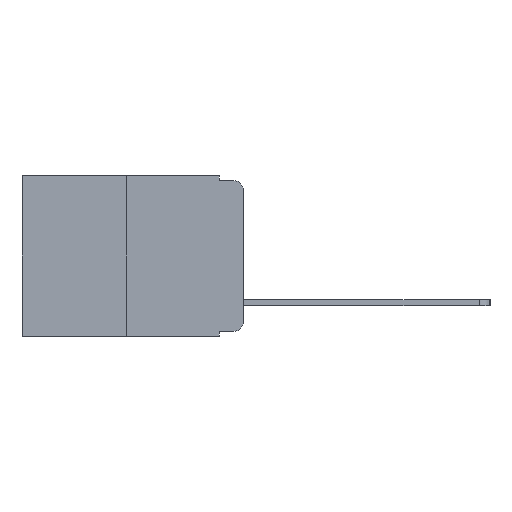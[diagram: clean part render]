
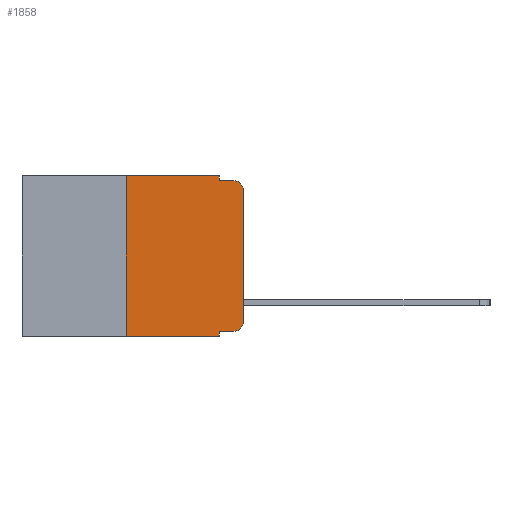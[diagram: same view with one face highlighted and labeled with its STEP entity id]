
A CAD part, left-side view. The second image highlights one B-rep face of the part: STEP entity #1858.
In plain terms, the highlighted planar face has unit normal (-1, 0, 0).
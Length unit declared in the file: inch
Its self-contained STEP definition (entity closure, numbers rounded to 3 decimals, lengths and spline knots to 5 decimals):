
#98 = DIRECTION ( 'NONE',  ( 0., 0., 1. ) ) ;
#257 = DIRECTION ( 'NONE',  ( 0., 0., -1. ) ) ;
#372 = CIRCLE ( 'NONE', #8661, 0.02 ) ;
#564 = DIRECTION ( 'NONE',  ( 0., 0., -1. ) ) ;
#1256 = EDGE_CURVE ( 'NONE', #14005, #2624, #5090, .T. ) ;
#1356 = DIRECTION ( 'NONE',  ( 0., 0., -1. ) ) ;
#1439 = CARTESIAN_POINT ( 'NONE',  ( 0., 0., -0.313 ) ) ;
#1517 = VERTEX_POINT ( 'NONE', #8939 ) ;
#1563 = AXIS2_PLACEMENT_3D ( 'NONE', #9882, #9736, #1356 ) ;
#1858 = ADVANCED_FACE ( 'NONE', ( #3646 ), #2925, .F. ) ;
#1863 = CIRCLE ( 'NONE', #1563, 0.02 ) ;
#1939 = AXIS2_PLACEMENT_3D ( 'NONE', #11509, #14015, #564 ) ;
#2019 = DIRECTION ( 'NONE',  ( 0., -1., 0. ) ) ;
#2057 = VECTOR ( 'NONE', #257, 39.37008 ) ;
#2066 = EDGE_CURVE ( 'NONE', #2624, #2464, #7637, .T. ) ;
#2093 = VERTEX_POINT ( 'NONE', #12054 ) ;
#2464 = VERTEX_POINT ( 'NONE', #9308 ) ;
#2624 = VERTEX_POINT ( 'NONE', #13218 ) ;
#2839 = EDGE_CURVE ( 'NONE', #8152, #2464, #1863, .T. ) ;
#2925 = PLANE ( 'NONE',  #1939 ) ;
#3014 = VERTEX_POINT ( 'NONE', #9591 ) ;
#3192 = DIRECTION ( 'NONE',  ( -1., 0., 0. ) ) ;
#3607 = EDGE_CURVE ( 'NONE', #10266, #8152, #13814, .T. ) ;
#3646 = FACE_OUTER_BOUND ( 'NONE', #8747, .T. ) ;
#4068 = VECTOR ( 'NONE', #10616, 39.37008 ) ;
#4423 = ORIENTED_EDGE ( 'NONE', *, *, #11782, .T. ) ;
#4473 = ORIENTED_EDGE ( 'NONE', *, *, #2839, .T. ) ;
#4500 = ORIENTED_EDGE ( 'NONE', *, *, #13169, .F. ) ;
#5040 = EDGE_CURVE ( 'NONE', #2093, #14005, #5875, .T. ) ;
#5090 = LINE ( 'NONE', #5540, #2057 ) ;
#5299 = CARTESIAN_POINT ( 'NONE',  ( 0., 0., -0.03 ) ) ;
#5330 = ORIENTED_EDGE ( 'NONE', *, *, #5575, .T. ) ;
#5540 = CARTESIAN_POINT ( 'NONE',  ( 0., 0.051, 0. ) ) ;
#5575 = EDGE_CURVE ( 'NONE', #6761, #11170, #6533, .T. ) ;
#5875 = LINE ( 'NONE', #13402, #11156 ) ;
#5907 = CARTESIAN_POINT ( 'NONE',  ( 0., 0.25, 0. ) ) ;
#5914 = VECTOR ( 'NONE', #98, 39.37008 ) ;
#6533 = LINE ( 'NONE', #6956, #13928 ) ;
#6761 = VERTEX_POINT ( 'NONE', #13907 ) ;
#6956 = CARTESIAN_POINT ( 'NONE',  ( 0., 0.473, -0.343 ) ) ;
#6981 = CARTESIAN_POINT ( 'NONE',  ( 0., 0.051, 0. ) ) ;
#7002 = DIRECTION ( 'NONE',  ( 0., -1., 0. ) ) ;
#7435 = ORIENTED_EDGE ( 'NONE', *, *, #3607, .T. ) ;
#7584 = ORIENTED_EDGE ( 'NONE', *, *, #12491, .T. ) ;
#7637 = LINE ( 'NONE', #9596, #10045 ) ;
#7987 = DIRECTION ( 'NONE',  ( 0., 0., -1. ) ) ;
#8010 = ORIENTED_EDGE ( 'NONE', *, *, #13865, .F. ) ;
#8152 = VERTEX_POINT ( 'NONE', #5299 ) ;
#8364 = LINE ( 'NONE', #5907, #5914 ) ;
#8661 = AXIS2_PLACEMENT_3D ( 'NONE', #9621, #3192, #10726 ) ;
#8747 = EDGE_LOOP ( 'NONE', ( #7435, #4473, #11200, #10667, #9492, #8010, #5330, #4500, #7584, #4423 ) ) ;
#8939 = CARTESIAN_POINT ( 'NONE',  ( 0., 0.02, -0.333 ) ) ;
#9308 = CARTESIAN_POINT ( 'NONE',  ( 0., 0.02, -0.01 ) ) ;
#9492 = ORIENTED_EDGE ( 'NONE', *, *, #5040, .F. ) ;
#9516 = CARTESIAN_POINT ( 'NONE',  ( 0., 0.051, -0.333 ) ) ;
#9581 = DIRECTION ( 'NONE',  ( 0., -1., 0. ) ) ;
#9591 = CARTESIAN_POINT ( 'NONE',  ( 0., 0.051, -0.333 ) ) ;
#9596 = CARTESIAN_POINT ( 'NONE',  ( 0., 0.051, -0.01 ) ) ;
#9621 = CARTESIAN_POINT ( 'NONE',  ( 0., 0.02, -0.313 ) ) ;
#9736 = DIRECTION ( 'NONE',  ( -1., 0., 0. ) ) ;
#9882 = CARTESIAN_POINT ( 'NONE',  ( 0., 0.02, -0.03 ) ) ;
#10034 = VECTOR ( 'NONE', #7987, 39.37008 ) ;
#10045 = VECTOR ( 'NONE', #9581, 39.37008 ) ;
#10266 = VERTEX_POINT ( 'NONE', #1439 ) ;
#10323 = CARTESIAN_POINT ( 'NONE',  ( 0., 0.051, 0. ) ) ;
#10616 = DIRECTION ( 'NONE',  ( 0., -1., 0. ) ) ;
#10667 = ORIENTED_EDGE ( 'NONE', *, *, #1256, .F. ) ;
#10726 = DIRECTION ( 'NONE',  ( 0., 0., -1. ) ) ;
#10959 = CARTESIAN_POINT ( 'NONE',  ( 0., 0.051, -0.343 ) ) ;
#11156 = VECTOR ( 'NONE', #7002, 39.37008 ) ;
#11170 = VERTEX_POINT ( 'NONE', #10959 ) ;
#11200 = ORIENTED_EDGE ( 'NONE', *, *, #2066, .F. ) ;
#11509 = CARTESIAN_POINT ( 'NONE',  ( 0., 0.473, 0. ) ) ;
#11782 = EDGE_CURVE ( 'NONE', #1517, #10266, #372, .T. ) ;
#11938 = CARTESIAN_POINT ( 'NONE',  ( 0., 0., 0. ) ) ;
#12021 = DIRECTION ( 'NONE',  ( 0., 0., 1. ) ) ;
#12054 = CARTESIAN_POINT ( 'NONE',  ( 0., 0.25, 0. ) ) ;
#12491 = EDGE_CURVE ( 'NONE', #3014, #1517, #13211, .T. ) ;
#13169 = EDGE_CURVE ( 'NONE', #3014, #11170, #13185, .T. ) ;
#13185 = LINE ( 'NONE', #6981, #10034 ) ;
#13211 = LINE ( 'NONE', #9516, #4068 ) ;
#13218 = CARTESIAN_POINT ( 'NONE',  ( 0., 0.051, -0.01 ) ) ;
#13402 = CARTESIAN_POINT ( 'NONE',  ( 0., 0.473, 0. ) ) ;
#13489 = VECTOR ( 'NONE', #12021, 39.37008 ) ;
#13814 = LINE ( 'NONE', #11938, #13489 ) ;
#13865 = EDGE_CURVE ( 'NONE', #6761, #2093, #8364, .T. ) ;
#13907 = CARTESIAN_POINT ( 'NONE',  ( 0., 0.25, -0.343 ) ) ;
#13928 = VECTOR ( 'NONE', #2019, 39.37008 ) ;
#14005 = VERTEX_POINT ( 'NONE', #10323 ) ;
#14015 = DIRECTION ( 'NONE',  ( 1., 0., 0. ) ) ;
